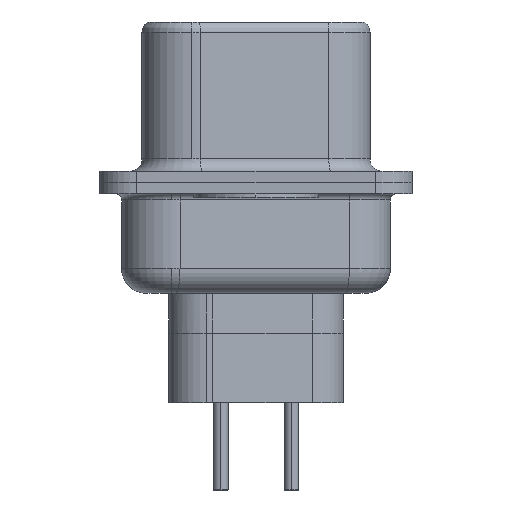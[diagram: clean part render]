
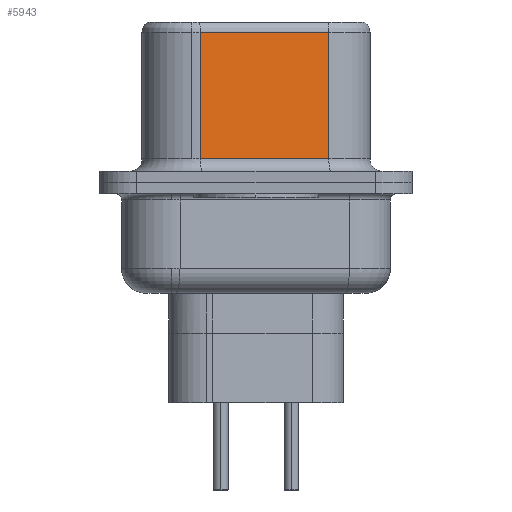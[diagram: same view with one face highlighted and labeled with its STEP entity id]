
A CAD part, left-side view. The second image highlights one B-rep face of the part: STEP entity #5943.
In plain terms, the highlighted planar face has unit normal (-0.985, -0.174, 0).
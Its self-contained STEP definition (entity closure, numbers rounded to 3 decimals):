
#466 = EDGE_CURVE ( 'NONE', #4171, #7793, #8361, .T. ) ;
#815 = CARTESIAN_POINT ( 'NONE',  ( 4.575, -2.927, 6.02 ) ) ;
#1604 = CARTESIAN_POINT ( 'NONE',  ( 4.575, -2.927, 6.52 ) ) ;
#2830 = VECTOR ( 'NONE', #19176, 1000. ) ;
#3811 = DIRECTION ( 'NONE',  ( 0., 0., -1. ) ) ;
#3908 = DIRECTION ( 'NONE',  ( -0.174, 0.985, 0. ) ) ;
#3971 = VECTOR ( 'NONE', #3811, 1000. ) ;
#4072 = VECTOR ( 'NONE', #12684, 1000. ) ;
#4171 = VERTEX_POINT ( 'NONE', #7799 ) ;
#4702 = PLANE ( 'NONE',  #6913 ) ;
#4815 = DIRECTION ( 'NONE',  ( -0.174, 0.985, 0. ) ) ;
#5238 = ORIENTED_EDGE ( 'NONE', *, *, #9819, .T. ) ;
#5943 = ADVANCED_FACE ( 'NONE', ( #20722 ), #4702, .F. ) ;
#6268 = CARTESIAN_POINT ( 'NONE',  ( 4.575, -2.927, 0.95 ) ) ;
#6316 = LINE ( 'NONE', #14274, #4072 ) ;
#6913 = AXIS2_PLACEMENT_3D ( 'NONE', #1604, #20929, #4815 ) ;
#7793 = VERTEX_POINT ( 'NONE', #19841 ) ;
#7799 = CARTESIAN_POINT ( 'NONE',  ( 3.665, 2.233, 6.02 ) ) ;
#8361 = LINE ( 'NONE', #13231, #3971 ) ;
#9015 = VERTEX_POINT ( 'NONE', #15542 ) ;
#9819 = EDGE_CURVE ( 'NONE', #7793, #11544, #6316, .T. ) ;
#10594 = EDGE_CURVE ( 'NONE', #9015, #4171, #12358, .T. ) ;
#11128 = ORIENTED_EDGE ( 'NONE', *, *, #10594, .T. ) ;
#11544 = VERTEX_POINT ( 'NONE', #6268 ) ;
#12358 = LINE ( 'NONE', #815, #13177 ) ;
#12684 = DIRECTION ( 'NONE',  ( 0.174, -0.985, 0. ) ) ;
#13177 = VECTOR ( 'NONE', #3908, 1000. ) ;
#13231 = CARTESIAN_POINT ( 'NONE',  ( 3.665, 2.233, 6.52 ) ) ;
#13981 = EDGE_CURVE ( 'NONE', #9015, #11544, #16002, .T. ) ;
#14151 = EDGE_LOOP ( 'NONE', ( #17598, #11128, #18381, #5238 ) ) ;
#14274 = CARTESIAN_POINT ( 'NONE',  ( 4.575, -2.927, 0.95 ) ) ;
#15542 = CARTESIAN_POINT ( 'NONE',  ( 4.575, -2.927, 6.02 ) ) ;
#16002 = LINE ( 'NONE', #16310, #2830 ) ;
#16310 = CARTESIAN_POINT ( 'NONE',  ( 4.575, -2.927, 6.52 ) ) ;
#17598 = ORIENTED_EDGE ( 'NONE', *, *, #13981, .F. ) ;
#18381 = ORIENTED_EDGE ( 'NONE', *, *, #466, .T. ) ;
#19176 = DIRECTION ( 'NONE',  ( 0., 0., -1. ) ) ;
#19841 = CARTESIAN_POINT ( 'NONE',  ( 3.665, 2.233, 0.95 ) ) ;
#20722 = FACE_OUTER_BOUND ( 'NONE', #14151, .T. ) ;
#20929 = DIRECTION ( 'NONE',  ( 0.985, 0.174, 0. ) ) ;
